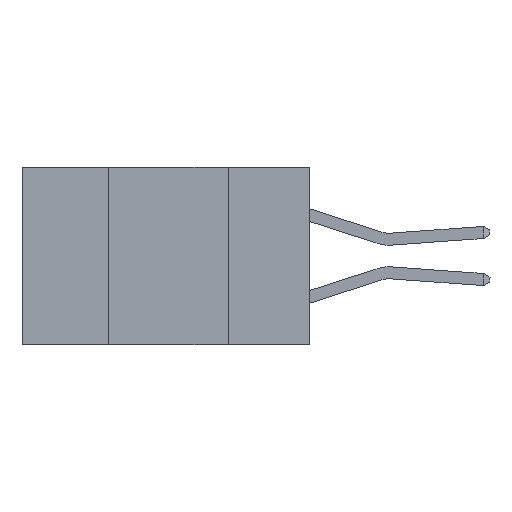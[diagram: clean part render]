
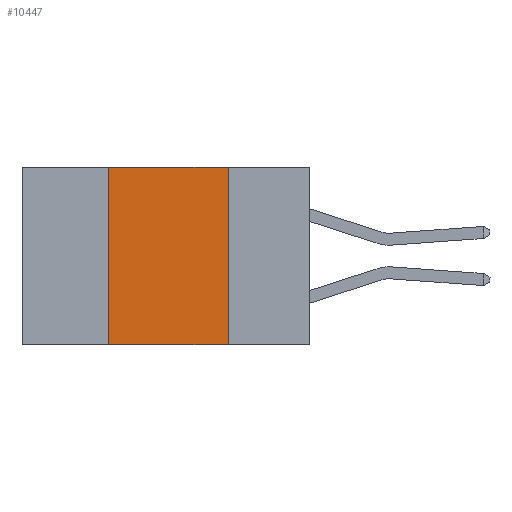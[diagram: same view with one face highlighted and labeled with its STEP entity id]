
A CAD part, left-side view. The second image highlights one B-rep face of the part: STEP entity #10447.
In plain terms, the highlighted planar face has unit normal (-1, 0, 0).
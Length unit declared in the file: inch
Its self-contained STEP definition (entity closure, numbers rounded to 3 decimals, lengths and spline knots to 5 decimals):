
#17 = VECTOR ( 'NONE', #15399, 39.37008 ) ;
#328 = VECTOR ( 'NONE', #6517, 39.37008 ) ;
#625 = ORIENTED_EDGE ( 'NONE', *, *, #7986, .F. ) ;
#1163 = DIRECTION ( 'NONE',  ( 1., 0., 0. ) ) ;
#1569 = CARTESIAN_POINT ( 'NONE',  ( 0., 0.17, 0. ) ) ;
#1963 = CARTESIAN_POINT ( 'NONE',  ( 0., 0.42, 0. ) ) ;
#2359 = DIRECTION ( 'NONE',  ( 0., 0., -1. ) ) ;
#2549 = ORIENTED_EDGE ( 'NONE', *, *, #4997, .F. ) ;
#3029 = LINE ( 'NONE', #14741, #7649 ) ;
#3033 = VERTEX_POINT ( 'NONE', #1569 ) ;
#3782 = DIRECTION ( 'NONE',  ( 0., -1., 0. ) ) ;
#4783 = PLANE ( 'NONE',  #10621 ) ;
#4895 = CARTESIAN_POINT ( 'NONE',  ( 0., 0.6, 0. ) ) ;
#4997 = EDGE_CURVE ( 'NONE', #3033, #6122, #13029, .T. ) ;
#5704 = ORIENTED_EDGE ( 'NONE', *, *, #15581, .F. ) ;
#5899 = VERTEX_POINT ( 'NONE', #6524 ) ;
#5966 = CARTESIAN_POINT ( 'NONE',  ( 0., 0.17, -0.37 ) ) ;
#6122 = VERTEX_POINT ( 'NONE', #5966 ) ;
#6355 = CARTESIAN_POINT ( 'NONE',  ( 0., 0.6, 0. ) ) ;
#6445 = VECTOR ( 'NONE', #8568, 39.37008 ) ;
#6517 = DIRECTION ( 'NONE',  ( 0., -1., 0. ) ) ;
#6524 = CARTESIAN_POINT ( 'NONE',  ( 0., 0.42, 0. ) ) ;
#6748 = LINE ( 'NONE', #1963, #17 ) ;
#6856 = LINE ( 'NONE', #6355, #328 ) ;
#7649 = VECTOR ( 'NONE', #3782, 39.37008 ) ;
#7986 = EDGE_CURVE ( 'NONE', #8104, #5899, #6748, .T. ) ;
#8104 = VERTEX_POINT ( 'NONE', #9558 ) ;
#8568 = DIRECTION ( 'NONE',  ( 0., 0., -1. ) ) ;
#8771 = EDGE_LOOP ( 'NONE', ( #2549, #5704, #625, #15097 ) ) ;
#9558 = CARTESIAN_POINT ( 'NONE',  ( 0., 0.42, -0.37 ) ) ;
#10447 = ADVANCED_FACE ( 'NONE', ( #12078 ), #4783, .F. ) ;
#10621 = AXIS2_PLACEMENT_3D ( 'NONE', #4895, #1163, #2359 ) ;
#12078 = FACE_OUTER_BOUND ( 'NONE', #8771, .T. ) ;
#12262 = CARTESIAN_POINT ( 'NONE',  ( 0., 0.17, 0. ) ) ;
#13029 = LINE ( 'NONE', #12262, #6445 ) ;
#14741 = CARTESIAN_POINT ( 'NONE',  ( 0., 0.6, -0.37 ) ) ;
#14948 = EDGE_CURVE ( 'NONE', #8104, #6122, #3029, .T. ) ;
#15097 = ORIENTED_EDGE ( 'NONE', *, *, #14948, .T. ) ;
#15399 = DIRECTION ( 'NONE',  ( 0., 0., 1. ) ) ;
#15581 = EDGE_CURVE ( 'NONE', #5899, #3033, #6856, .T. ) ;
